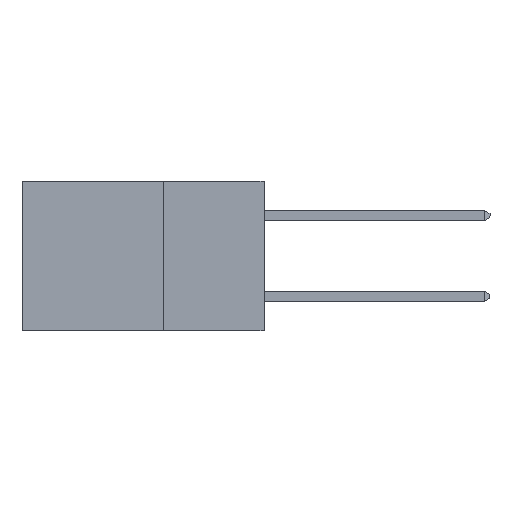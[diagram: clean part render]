
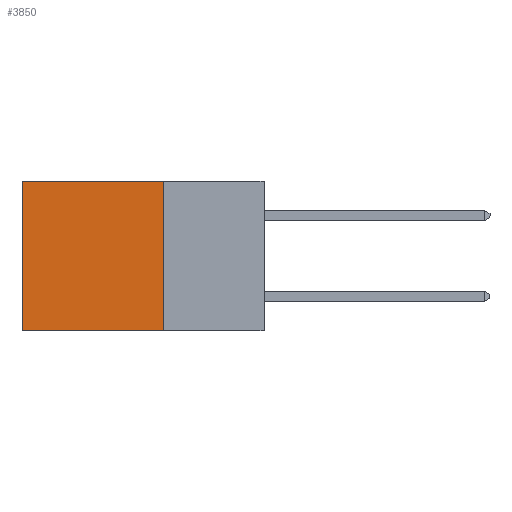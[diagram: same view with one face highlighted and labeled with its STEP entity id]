
A CAD part, left-side view. The second image highlights one B-rep face of the part: STEP entity #3850.
In plain terms, the highlighted planar face has unit normal (-1, 0, 0).
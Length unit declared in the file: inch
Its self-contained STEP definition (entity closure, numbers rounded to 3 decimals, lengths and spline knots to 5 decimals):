
#139 = CARTESIAN_POINT ( 'NONE',  ( 0.298, 0.6, -0.37 ) ) ;
#355 = EDGE_CURVE ( 'NONE', #8959, #9769, #11963, .T. ) ;
#736 = ORIENTED_EDGE ( 'NONE', *, *, #355, .F. ) ;
#775 = CARTESIAN_POINT ( 'NONE',  ( 0.298, 0.6, 0. ) ) ;
#1392 = ORIENTED_EDGE ( 'NONE', *, *, #12587, .F. ) ;
#1403 = ORIENTED_EDGE ( 'NONE', *, *, #5238, .T. ) ;
#1823 = VECTOR ( 'NONE', #8417, 39.37008 ) ;
#2268 = CARTESIAN_POINT ( 'NONE',  ( 0.298, 0.6, 0. ) ) ;
#3118 = FACE_OUTER_BOUND ( 'NONE', #6810, .T. ) ;
#3519 = DIRECTION ( 'NONE',  ( 1., 0., 0. ) ) ;
#3850 = ADVANCED_FACE ( 'NONE', ( #3118 ), #5252, .F. ) ;
#5106 = CARTESIAN_POINT ( 'NONE',  ( 0.298, 0.25, -0.37 ) ) ;
#5238 = EDGE_CURVE ( 'NONE', #10073, #8780, #10981, .T. ) ;
#5252 = PLANE ( 'NONE',  #8058 ) ;
#5270 = DIRECTION ( 'NONE',  ( 0., 0., -1. ) ) ;
#5355 = CARTESIAN_POINT ( 'NONE',  ( 0.298, 0.25, 0. ) ) ;
#5477 = VECTOR ( 'NONE', #8362, 39.37008 ) ;
#5726 = CARTESIAN_POINT ( 'NONE',  ( 0.298, 0.25, 0. ) ) ;
#6516 = VECTOR ( 'NONE', #10650, 39.37008 ) ;
#6810 = EDGE_LOOP ( 'NONE', ( #11201, #736, #1392, #1403 ) ) ;
#7215 = EDGE_CURVE ( 'NONE', #8780, #9769, #9375, .T. ) ;
#8058 = AXIS2_PLACEMENT_3D ( 'NONE', #5355, #3519, #5270 ) ;
#8362 = DIRECTION ( 'NONE',  ( 0., 1., 0. ) ) ;
#8405 = CARTESIAN_POINT ( 'NONE',  ( 0.298, 0.25, 0. ) ) ;
#8417 = DIRECTION ( 'NONE',  ( 0., 0., -1. ) ) ;
#8780 = VERTEX_POINT ( 'NONE', #775 ) ;
#8959 = VERTEX_POINT ( 'NONE', #5106 ) ;
#9296 = VECTOR ( 'NONE', #10251, 39.37008 ) ;
#9375 = LINE ( 'NONE', #2268, #1823 ) ;
#9604 = CARTESIAN_POINT ( 'NONE',  ( 0.298, 0.25, 0. ) ) ;
#9769 = VERTEX_POINT ( 'NONE', #139 ) ;
#10073 = VERTEX_POINT ( 'NONE', #5726 ) ;
#10251 = DIRECTION ( 'NONE',  ( 0., 1., 0. ) ) ;
#10650 = DIRECTION ( 'NONE',  ( 0., 0., -1. ) ) ;
#10941 = CARTESIAN_POINT ( 'NONE',  ( 0.298, 0.25, -0.37 ) ) ;
#10981 = LINE ( 'NONE', #8405, #5477 ) ;
#11201 = ORIENTED_EDGE ( 'NONE', *, *, #7215, .T. ) ;
#11902 = LINE ( 'NONE', #9604, #6516 ) ;
#11963 = LINE ( 'NONE', #10941, #9296 ) ;
#12587 = EDGE_CURVE ( 'NONE', #10073, #8959, #11902, .T. ) ;
